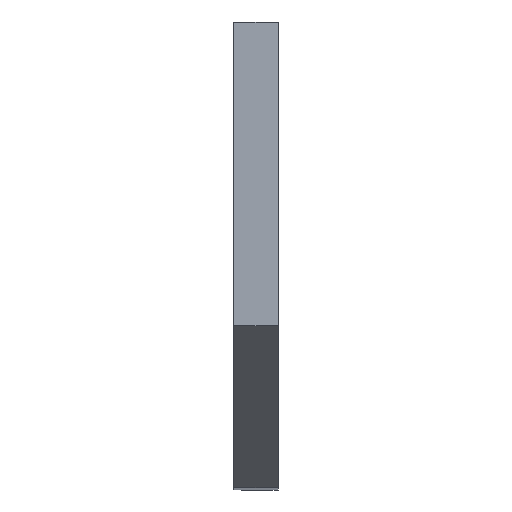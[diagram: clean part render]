
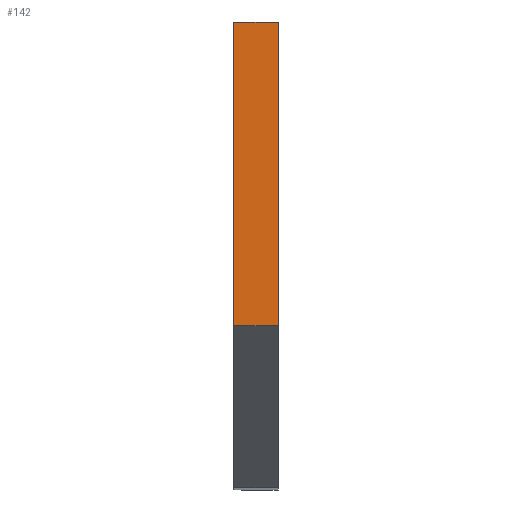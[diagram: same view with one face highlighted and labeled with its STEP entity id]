
A CAD part, top view. The second image highlights one B-rep face of the part: STEP entity #142.
In plain terms, the highlighted planar face has unit normal (0, 0, 1).
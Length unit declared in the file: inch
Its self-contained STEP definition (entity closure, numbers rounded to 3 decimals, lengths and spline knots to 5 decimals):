
#59 = ORIENTED_EDGE ( 'NONE', *, *, #1217, .T. ) ;
#86 = VERTEX_POINT ( 'NONE', #746 ) ;
#142 = ADVANCED_FACE ( 'NONE', ( #914 ), #965, .F. ) ;
#193 = CARTESIAN_POINT ( 'NONE',  ( 0.125, 0., 0. ) ) ;
#259 = VERTEX_POINT ( 'NONE', #1042 ) ;
#353 = LINE ( 'NONE', #1173, #964 ) ;
#361 = DIRECTION ( 'NONE',  ( -1., 0., 0. ) ) ;
#421 = CARTESIAN_POINT ( 'NONE',  ( 0.125, 0.457, 0. ) ) ;
#434 = EDGE_LOOP ( 'NONE', ( #1138, #755, #481, #59 ) ) ;
#474 = VECTOR ( 'NONE', #1362, 39.37008 ) ;
#481 = ORIENTED_EDGE ( 'NONE', *, *, #1371, .F. ) ;
#486 = VECTOR ( 'NONE', #1354, 39.37008 ) ;
#495 = CARTESIAN_POINT ( 'NONE',  ( 0., 1.316, 0. ) ) ;
#658 = CARTESIAN_POINT ( 'NONE',  ( 0.125, 0.457, 0. ) ) ;
#746 = CARTESIAN_POINT ( 'NONE',  ( 0., 0.457, 0. ) ) ;
#755 = ORIENTED_EDGE ( 'NONE', *, *, #1350, .F. ) ;
#777 = LINE ( 'NONE', #1128, #474 ) ;
#866 = VERTEX_POINT ( 'NONE', #495 ) ;
#884 = DIRECTION ( 'NONE',  ( 0., -1., 0. ) ) ;
#914 = FACE_OUTER_BOUND ( 'NONE', #434, .T. ) ;
#964 = VECTOR ( 'NONE', #361, 39.37008 ) ;
#965 = PLANE ( 'NONE',  #985 ) ;
#978 = DIRECTION ( 'NONE',  ( 0., 0., -1. ) ) ;
#979 = VECTOR ( 'NONE', #884, 39.37008 ) ;
#984 = EDGE_CURVE ( 'NONE', #866, #86, #777, .T. ) ;
#985 = AXIS2_PLACEMENT_3D ( 'NONE', #1211, #978, #1009 ) ;
#1009 = DIRECTION ( 'NONE',  ( 0., 1., 0. ) ) ;
#1042 = CARTESIAN_POINT ( 'NONE',  ( 0.125, 1.316, 0. ) ) ;
#1128 = CARTESIAN_POINT ( 'NONE',  ( 0., 0., 0. ) ) ;
#1138 = ORIENTED_EDGE ( 'NONE', *, *, #984, .T. ) ;
#1173 = CARTESIAN_POINT ( 'NONE',  ( 0.125, 1.316, 0. ) ) ;
#1211 = CARTESIAN_POINT ( 'NONE',  ( 0.125, 0., 0. ) ) ;
#1217 = EDGE_CURVE ( 'NONE', #259, #866, #353, .T. ) ;
#1296 = LINE ( 'NONE', #193, #979 ) ;
#1333 = LINE ( 'NONE', #658, #486 ) ;
#1350 = EDGE_CURVE ( 'NONE', #1392, #86, #1333, .T. ) ;
#1354 = DIRECTION ( 'NONE',  ( -1., 0., 0. ) ) ;
#1362 = DIRECTION ( 'NONE',  ( 0., -1., 0. ) ) ;
#1371 = EDGE_CURVE ( 'NONE', #259, #1392, #1296, .T. ) ;
#1392 = VERTEX_POINT ( 'NONE', #421 ) ;
